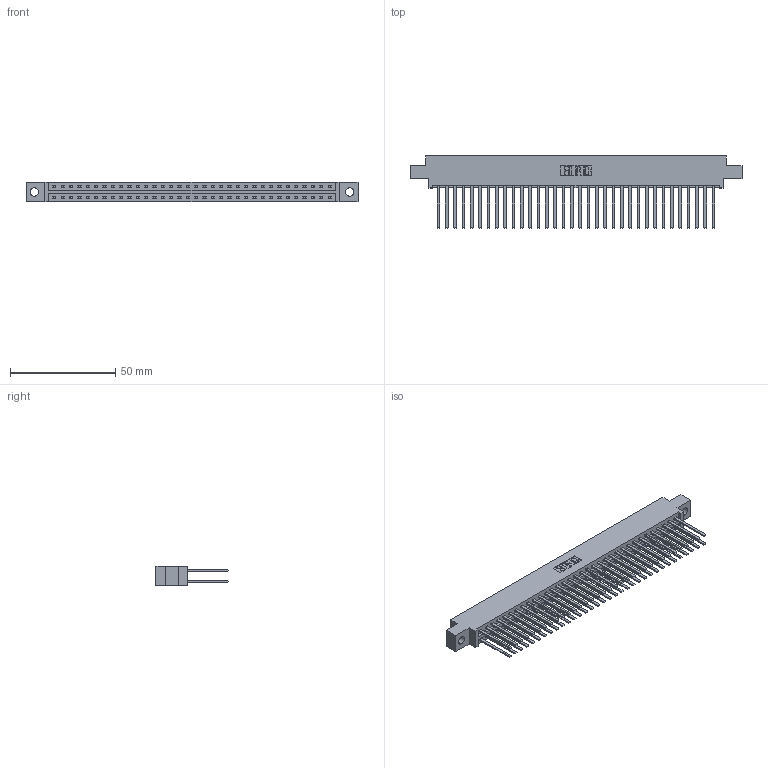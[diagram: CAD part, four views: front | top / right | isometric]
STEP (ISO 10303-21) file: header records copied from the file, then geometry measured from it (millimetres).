
FILE_DESCRIPTION (( 'STEP AP203' ), '1' );
FILE_NAME ('387-068-544-804.STEP', '2019-10-19T21:28:10', ( '' ), ( '' ), 'SwSTEP 2.0', 'SolidWorks 2016', '' );
FILE_SCHEMA (( 'CONFIG_CONTROL_DESIGN' ));
Length unit declared in the file: inch
Products named in the file (3): 337 Part_0.170 Offset - 0.156 Dia-TH; 387-068-544-804; 345-292-001_345-293-144
Assembly tree (69 placements, depth 2):
  387-068-544-804
    337 Part_0.170 Offset - 0.156 Dia-TH
    345-292-001_345-293-144  x68
Bounding box: 157.73 x 34.3 x 9.4 mm (x, y, z)
Volume: 17264.6 mm3; surface area: 22459.2 mm2
Topology: 69 solids, 69 shells, 3382 faces, 10047 edges, 6606 vertices
Faces by surface type: plane 2386, cylinder 996
Entity records: 27347 total; most frequent: CARTESIAN_POINT 4614, ORIENTED_EDGE 4550, DIRECTION 3935, EDGE_CURVE 2275, LINE 2151, VECTOR 2151, VERTEX_POINT 1514, AXIS2_PLACEMENT_3D 892
